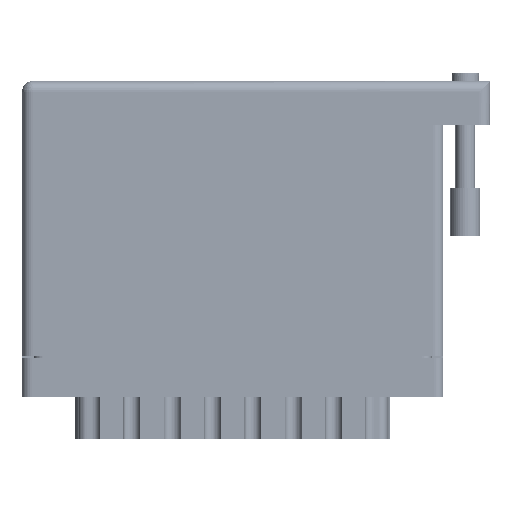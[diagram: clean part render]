
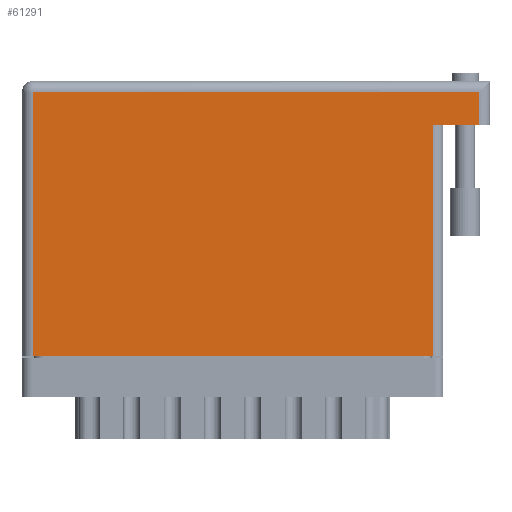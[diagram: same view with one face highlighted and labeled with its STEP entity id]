
A CAD part, front view. The second image highlights one B-rep face of the part: STEP entity #61291.
In plain terms, the highlighted face is planar.
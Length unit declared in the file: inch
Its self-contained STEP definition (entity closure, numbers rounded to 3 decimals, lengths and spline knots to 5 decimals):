
#2639 = DIRECTION ( 'NONE',  ( 1., 0., 0. ) ) ;
#2939 = DIRECTION ( 'NONE',  ( 0., -1., 0. ) ) ;
#2980 = ORIENTED_EDGE ( 'NONE', *, *, #72505, .T. ) ;
#3709 = CARTESIAN_POINT ( 'NONE',  ( 0.07, 0., 0. ) ) ;
#6766 = EDGE_CURVE ( 'NONE', #11983, #12869, #23419, .T. ) ;
#8283 = ORIENTED_EDGE ( 'NONE', *, *, #27106, .T. ) ;
#9136 = DIRECTION ( 'NONE',  ( 0., 1., 0. ) ) ;
#9161 = VERTEX_POINT ( 'NONE', #41943 ) ;
#10921 = VERTEX_POINT ( 'NONE', #37948 ) ;
#11983 = VERTEX_POINT ( 'NONE', #62586 ) ;
#12869 = VERTEX_POINT ( 'NONE', #31919 ) ;
#13483 = LINE ( 'NONE', #37786, #14989 ) ;
#13787 = VERTEX_POINT ( 'NONE', #26990 ) ;
#14989 = VECTOR ( 'NONE', #2639, 39.37008 ) ;
#15922 = EDGE_LOOP ( 'NONE', ( #34163, #8283, #24803, #2980, #35654, #32346 ) ) ;
#18825 = DIRECTION ( 'NONE',  ( 0., 0., -1. ) ) ;
#21852 = LINE ( 'NONE', #56230, #61737 ) ;
#22653 = CARTESIAN_POINT ( 'NONE',  ( 0., 1.705, 0. ) ) ;
#23419 = LINE ( 'NONE', #22653, #65683 ) ;
#24803 = ORIENTED_EDGE ( 'NONE', *, *, #58462, .F. ) ;
#26990 = CARTESIAN_POINT ( 'NONE',  ( 0.07, 0., 0. ) ) ;
#27106 = EDGE_CURVE ( 'NONE', #56482, #9161, #53688, .T. ) ;
#27471 = AXIS2_PLACEMENT_3D ( 'NONE', #73255, #18825, #60895 ) ;
#31919 = CARTESIAN_POINT ( 'NONE',  ( 0.07, 1.705, 0. ) ) ;
#32346 = ORIENTED_EDGE ( 'NONE', *, *, #68283, .T. ) ;
#33051 = LINE ( 'NONE', #3709, #54015 ) ;
#34163 = ORIENTED_EDGE ( 'NONE', *, *, #48946, .T. ) ;
#35654 = ORIENTED_EDGE ( 'NONE', *, *, #6766, .T. ) ;
#37786 = CARTESIAN_POINT ( 'NONE',  ( 0., 0., 0. ) ) ;
#37948 = CARTESIAN_POINT ( 'NONE',  ( 2.948, 1.495, 0. ) ) ;
#41943 = CARTESIAN_POINT ( 'NONE',  ( 2.648, 1.495, 0. ) ) ;
#43133 = PLANE ( 'NONE',  #27471 ) ;
#46347 = CARTESIAN_POINT ( 'NONE',  ( 2.648, 1.495, 0. ) ) ;
#48946 = EDGE_CURVE ( 'NONE', #13787, #56482, #13483, .T. ) ;
#49293 = FACE_OUTER_BOUND ( 'NONE', #15922, .T. ) ;
#53312 = LINE ( 'NONE', #71484, #61375 ) ;
#53688 = LINE ( 'NONE', #46347, #59157 ) ;
#54015 = VECTOR ( 'NONE', #2939, 39.37008 ) ;
#56230 = CARTESIAN_POINT ( 'NONE',  ( 2.948, 1.775, 0. ) ) ;
#56482 = VERTEX_POINT ( 'NONE', #69918 ) ;
#58462 = EDGE_CURVE ( 'NONE', #10921, #9161, #53312, .T. ) ;
#59157 = VECTOR ( 'NONE', #71075, 39.37008 ) ;
#60895 = DIRECTION ( 'NONE',  ( -1., 0., 0. ) ) ;
#61291 = ADVANCED_FACE ( 'NONE', ( #49293 ), #43133, .F. ) ;
#61375 = VECTOR ( 'NONE', #73275, 39.37008 ) ;
#61737 = VECTOR ( 'NONE', #9136, 39.37008 ) ;
#62586 = CARTESIAN_POINT ( 'NONE',  ( 2.948, 1.705, 0. ) ) ;
#65107 = DIRECTION ( 'NONE',  ( -1., 0., 0. ) ) ;
#65683 = VECTOR ( 'NONE', #65107, 39.37008 ) ;
#68283 = EDGE_CURVE ( 'NONE', #12869, #13787, #33051, .T. ) ;
#69918 = CARTESIAN_POINT ( 'NONE',  ( 2.648, 0., 0. ) ) ;
#71075 = DIRECTION ( 'NONE',  ( 0., 1., 0. ) ) ;
#71484 = CARTESIAN_POINT ( 'NONE',  ( 3.018, 1.495, 0. ) ) ;
#72505 = EDGE_CURVE ( 'NONE', #10921, #11983, #21852, .T. ) ;
#73255 = CARTESIAN_POINT ( 'NONE',  ( 0., 1.775, 0. ) ) ;
#73275 = DIRECTION ( 'NONE',  ( -1., 0., 0. ) ) ;
